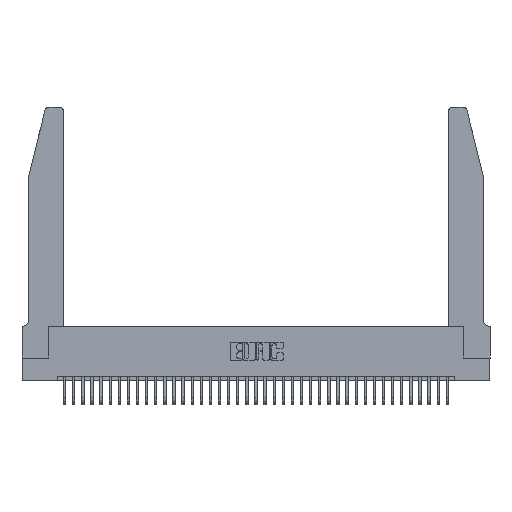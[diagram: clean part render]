
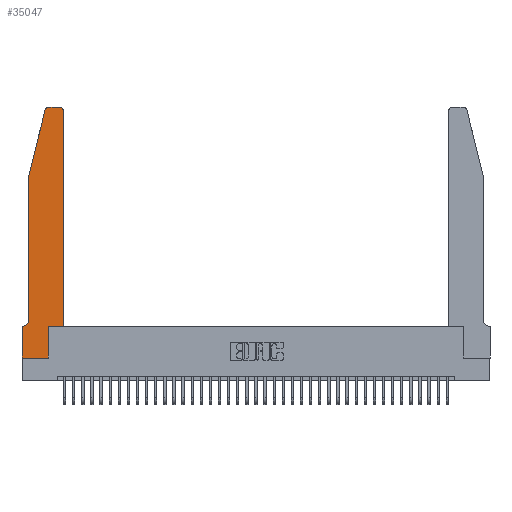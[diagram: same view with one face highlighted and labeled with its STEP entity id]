
A CAD part, top view. The second image highlights one B-rep face of the part: STEP entity #35047.
In plain terms, the highlighted planar face has unit normal (0, 0, 1).
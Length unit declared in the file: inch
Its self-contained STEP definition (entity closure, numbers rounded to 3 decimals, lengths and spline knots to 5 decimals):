
#470 = FACE_OUTER_BOUND ( 'NONE', #26174, .T. ) ;
#634 = VERTEX_POINT ( 'NONE', #22580 ) ;
#1182 = CARTESIAN_POINT ( 'NONE',  ( 0.4505, 0.35, 0.37 ) ) ;
#1216 = CARTESIAN_POINT ( 'NONE',  ( 0.284, 2.72, 0.37 ) ) ;
#1256 = CARTESIAN_POINT ( 'NONE',  ( 0.2865, 0.35, 0.37 ) ) ;
#2156 = LINE ( 'NONE', #5087, #16526 ) ;
#2483 = EDGE_CURVE ( 'NONE', #30691, #28742, #2156, .T. ) ;
#2532 = VERTEX_POINT ( 'NONE', #8255 ) ;
#2619 = VECTOR ( 'NONE', #33175, 39.37008 ) ;
#3188 = VERTEX_POINT ( 'NONE', #20052 ) ;
#3787 = DIRECTION ( 'NONE',  ( 0., 1., 0. ) ) ;
#4015 = ORIENTED_EDGE ( 'NONE', *, *, #10701, .T. ) ;
#4125 = DIRECTION ( 'NONE',  ( 1., 0., 0. ) ) ;
#4127 = VERTEX_POINT ( 'NONE', #23741 ) ;
#4918 = AXIS2_PLACEMENT_3D ( 'NONE', #32129, #15096, #35045 ) ;
#4955 = VECTOR ( 'NONE', #3787, 39.37008 ) ;
#5087 = CARTESIAN_POINT ( 'NONE',  ( 0.2605, 2.75, 0.37 ) ) ;
#5831 = CARTESIAN_POINT ( 'NONE',  ( 0.0055, 0.42, 0.37 ) ) ;
#5842 = EDGE_CURVE ( 'NONE', #30113, #23434, #17587, .T. ) ;
#5996 = DIRECTION ( 'NONE',  ( -1., 0., 0. ) ) ;
#6684 = VECTOR ( 'NONE', #31757, 39.37008 ) ;
#7048 = CARTESIAN_POINT ( 'NONE',  ( 0.4205, 2.72, 0.37 ) ) ;
#8098 = VECTOR ( 'NONE', #19631, 39.37008 ) ;
#8255 = CARTESIAN_POINT ( 'NONE',  ( 0.0755, 2., 0.37 ) ) ;
#8718 = ORIENTED_EDGE ( 'NONE', *, *, #16203, .T. ) ;
#8765 = DIRECTION ( 'NONE',  ( -1., 0., 0. ) ) ;
#8917 = CIRCLE ( 'NONE', #20043, 0.07 ) ;
#8967 = VECTOR ( 'NONE', #20969, 39.37008 ) ;
#9032 = CARTESIAN_POINT ( 'NONE',  ( 0., 0.35, 0.37 ) ) ;
#9160 = EDGE_CURVE ( 'NONE', #4127, #16309, #20167, .T. ) ;
#9521 = CARTESIAN_POINT ( 'NONE',  ( 0., 0., 0.37 ) ) ;
#9586 = CARTESIAN_POINT ( 'NONE',  ( 0.0755, 0.42, 0.37 ) ) ;
#9681 = CIRCLE ( 'NONE', #15771, 0.03 ) ;
#9885 = LINE ( 'NONE', #9521, #8967 ) ;
#9962 = DIRECTION ( 'NONE',  ( 1., 0., 0. ) ) ;
#10067 = ORIENTED_EDGE ( 'NONE', *, *, #19992, .T. ) ;
#10572 = CARTESIAN_POINT ( 'NONE',  ( 0.2865, 0.35, 0.37 ) ) ;
#10701 = EDGE_CURVE ( 'NONE', #28994, #30113, #8917, .T. ) ;
#11354 = CARTESIAN_POINT ( 'NONE',  ( 0.284, 2.75, 0.37 ) ) ;
#12174 = ORIENTED_EDGE ( 'NONE', *, *, #36515, .T. ) ;
#15052 = LINE ( 'NONE', #1182, #29289 ) ;
#15096 = DIRECTION ( 'NONE',  ( 0., 0., 1. ) ) ;
#15445 = EDGE_CURVE ( 'NONE', #634, #2532, #31695, .T. ) ;
#15533 = ORIENTED_EDGE ( 'NONE', *, *, #2483, .T. ) ;
#15771 = AXIS2_PLACEMENT_3D ( 'NONE', #1216, #21272, #4125 ) ;
#16203 = EDGE_CURVE ( 'NONE', #2532, #28994, #31196, .T. ) ;
#16309 = VERTEX_POINT ( 'NONE', #23818 ) ;
#16503 = DIRECTION ( 'NONE',  ( -1., 0., 0. ) ) ;
#16526 = VECTOR ( 'NONE', #16503, 39.37008 ) ;
#16670 = ORIENTED_EDGE ( 'NONE', *, *, #15445, .T. ) ;
#16677 = CIRCLE ( 'NONE', #26369, 0.03 ) ;
#17142 = VERTEX_POINT ( 'NONE', #10572 ) ;
#17468 = CARTESIAN_POINT ( 'NONE',  ( 0.0755, 2., 0.37 ) ) ;
#17587 = LINE ( 'NONE', #34472, #24278 ) ;
#18452 = DIRECTION ( 'NONE',  ( 0., 1., 0. ) ) ;
#18497 = LINE ( 'NONE', #1256, #31819 ) ;
#19631 = DIRECTION ( 'NONE',  ( -0.239, -0.971, 0. ) ) ;
#19947 = CARTESIAN_POINT ( 'NONE',  ( 0.0055, 0.35, 0.37 ) ) ;
#19992 = EDGE_CURVE ( 'NONE', #3188, #17142, #18497, .T. ) ;
#20043 = AXIS2_PLACEMENT_3D ( 'NONE', #5831, #25811, #8765 ) ;
#20052 = CARTESIAN_POINT ( 'NONE',  ( 0.2865, 0., 0.37 ) ) ;
#20167 = LINE ( 'NONE', #23790, #4955 ) ;
#20969 = DIRECTION ( 'NONE',  ( 1., 0., 0. ) ) ;
#21216 = EDGE_CURVE ( 'NONE', #28742, #634, #9681, .T. ) ;
#21272 = DIRECTION ( 'NONE',  ( 0., 0., 1. ) ) ;
#22580 = CARTESIAN_POINT ( 'NONE',  ( 0.25487, 2.72718, 0.37 ) ) ;
#23434 = VERTEX_POINT ( 'NONE', #9032 ) ;
#23741 = CARTESIAN_POINT ( 'NONE',  ( 0.4505, 0.35, 0.37 ) ) ;
#23790 = CARTESIAN_POINT ( 'NONE',  ( 0.4505, 0.35, 0.37 ) ) ;
#23818 = CARTESIAN_POINT ( 'NONE',  ( 0.4505, 2.72, 0.37 ) ) ;
#24278 = VECTOR ( 'NONE', #5996, 39.37008 ) ;
#24710 = ORIENTED_EDGE ( 'NONE', *, *, #32817, .T. ) ;
#25811 = DIRECTION ( 'NONE',  ( 0., 0., -1. ) ) ;
#26174 = EDGE_LOOP ( 'NONE', ( #15533, #28439, #16670, #8718, #4015, #28502, #12174, #36688, #10067, #24710, #26268, #34072 ) ) ;
#26268 = ORIENTED_EDGE ( 'NONE', *, *, #9160, .T. ) ;
#26369 = AXIS2_PLACEMENT_3D ( 'NONE', #7048, #27015, #9962 ) ;
#26409 = PLANE ( 'NONE',  #4918 ) ;
#27015 = DIRECTION ( 'NONE',  ( 0., 0., 1. ) ) ;
#27188 = VERTEX_POINT ( 'NONE', #28991 ) ;
#28224 = CARTESIAN_POINT ( 'NONE',  ( 0.0755, 2., 0.37 ) ) ;
#28439 = ORIENTED_EDGE ( 'NONE', *, *, #21216, .T. ) ;
#28502 = ORIENTED_EDGE ( 'NONE', *, *, #5842, .T. ) ;
#28742 = VERTEX_POINT ( 'NONE', #11354 ) ;
#28991 = CARTESIAN_POINT ( 'NONE',  ( 0., 0., 0.37 ) ) ;
#28994 = VERTEX_POINT ( 'NONE', #9586 ) ;
#29289 = VECTOR ( 'NONE', #35458, 39.37008 ) ;
#30113 = VERTEX_POINT ( 'NONE', #19947 ) ;
#30268 = CARTESIAN_POINT ( 'NONE',  ( 0., 0., 0.37 ) ) ;
#30691 = VERTEX_POINT ( 'NONE', #34748 ) ;
#30841 = EDGE_CURVE ( 'NONE', #16309, #30691, #16677, .T. ) ;
#31196 = LINE ( 'NONE', #17468, #6684 ) ;
#31695 = LINE ( 'NONE', #28224, #8098 ) ;
#31757 = DIRECTION ( 'NONE',  ( 0., -1., 0. ) ) ;
#31819 = VECTOR ( 'NONE', #18452, 39.37008 ) ;
#32129 = CARTESIAN_POINT ( 'NONE',  ( 0., 0.35, 0.37 ) ) ;
#32817 = EDGE_CURVE ( 'NONE', #17142, #4127, #15052, .T. ) ;
#33024 = LINE ( 'NONE', #30268, #2619 ) ;
#33175 = DIRECTION ( 'NONE',  ( 0., -1., 0. ) ) ;
#34072 = ORIENTED_EDGE ( 'NONE', *, *, #30841, .T. ) ;
#34472 = CARTESIAN_POINT ( 'NONE',  ( 0.0755, 0.35, 0.37 ) ) ;
#34748 = CARTESIAN_POINT ( 'NONE',  ( 0.4205, 2.75, 0.37 ) ) ;
#35045 = DIRECTION ( 'NONE',  ( 1., 0., 0. ) ) ;
#35047 = ADVANCED_FACE ( 'NONE', ( #470 ), #26409, .T. ) ;
#35458 = DIRECTION ( 'NONE',  ( 1., 0., 0. ) ) ;
#36341 = EDGE_CURVE ( 'NONE', #27188, #3188, #9885, .T. ) ;
#36515 = EDGE_CURVE ( 'NONE', #23434, #27188, #33024, .T. ) ;
#36688 = ORIENTED_EDGE ( 'NONE', *, *, #36341, .T. ) ;
